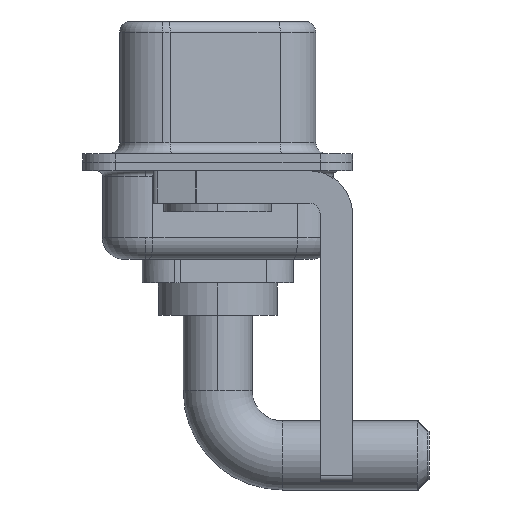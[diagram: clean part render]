
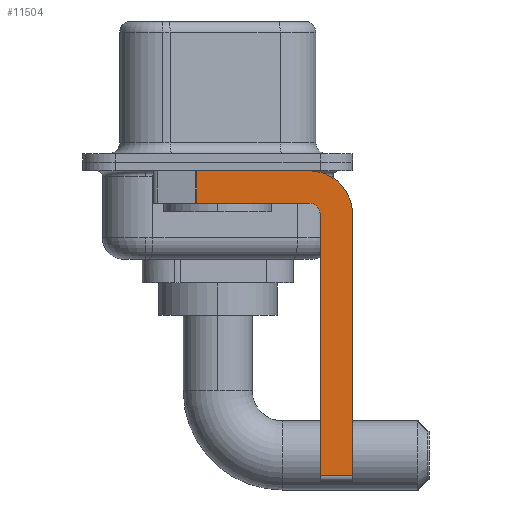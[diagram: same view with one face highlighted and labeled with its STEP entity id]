
A CAD part, left-side view. The second image highlights one B-rep face of the part: STEP entity #11504.
In plain terms, the highlighted planar face has unit normal (-1, 0, 0).
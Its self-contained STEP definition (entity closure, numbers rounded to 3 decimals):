
#90 = DIRECTION ( 'NONE',  ( 1., 0., 0. ) ) ;
#1001 = EDGE_CURVE ( 'NONE', #4662, #14181, #7622, .T. ) ;
#1189 = EDGE_CURVE ( 'NONE', #8029, #4716, #5484, .T. ) ;
#1194 = PLANE ( 'NONE',  #11478 ) ;
#1483 = CARTESIAN_POINT ( 'NONE',  ( -2.9, -4.25, -2.4 ) ) ;
#1550 = CARTESIAN_POINT ( 'NONE',  ( -2.9, -4.25, -2.4 ) ) ;
#1614 = CARTESIAN_POINT ( 'NONE',  ( -2.9, -4.25, -1.9 ) ) ;
#2068 = CARTESIAN_POINT ( 'NONE',  ( -2.9, 0.978, -1.9 ) ) ;
#2155 = CIRCLE ( 'NONE', #12160, 2. ) ;
#2481 = CARTESIAN_POINT ( 'NONE',  ( -2.9, 0.978, -0.4 ) ) ;
#3191 = CARTESIAN_POINT ( 'NONE',  ( -2.9, -4.75, -14.55 ) ) ;
#3294 = CARTESIAN_POINT ( 'NONE',  ( -2.9, -4.25, -0.4 ) ) ;
#3359 = CARTESIAN_POINT ( 'NONE',  ( -2.9, -4.75, -14.8 ) ) ;
#3788 = CARTESIAN_POINT ( 'NONE',  ( -2.9, -6.25, -2.4 ) ) ;
#3823 = EDGE_CURVE ( 'NONE', #8029, #11054, #7006, .T. ) ;
#3833 = CIRCLE ( 'NONE', #7467, 0.5 ) ;
#4075 = DIRECTION ( 'NONE',  ( 0., 1., 0. ) ) ;
#4662 = VERTEX_POINT ( 'NONE', #2481 ) ;
#4716 = VERTEX_POINT ( 'NONE', #11966 ) ;
#4869 = VERTEX_POINT ( 'NONE', #3788 ) ;
#4920 = EDGE_CURVE ( 'NONE', #11054, #5854, #3833, .T. ) ;
#4952 = EDGE_CURVE ( 'NONE', #4662, #5719, #13180, .T. ) ;
#5365 = ORIENTED_EDGE ( 'NONE', *, *, #5512, .F. ) ;
#5484 = LINE ( 'NONE', #8915, #11324 ) ;
#5512 = EDGE_CURVE ( 'NONE', #5854, #5719, #7645, .T. ) ;
#5719 = VERTEX_POINT ( 'NONE', #2068 ) ;
#5854 = VERTEX_POINT ( 'NONE', #13979 ) ;
#5855 = DIRECTION ( 'NONE',  ( 1., 0., 0. ) ) ;
#6202 = DIRECTION ( 'NONE',  ( 0., 0., -1. ) ) ;
#6381 = EDGE_CURVE ( 'NONE', #14181, #4869, #2155, .T. ) ;
#6847 = CARTESIAN_POINT ( 'NONE',  ( -2.9, -4.25, -2.4 ) ) ;
#7006 = LINE ( 'NONE', #3359, #7976 ) ;
#7363 = DIRECTION ( 'NONE',  ( 0., 0., -1. ) ) ;
#7467 = AXIS2_PLACEMENT_3D ( 'NONE', #1550, #11728, #14015 ) ;
#7622 = LINE ( 'NONE', #13445, #9769 ) ;
#7645 = LINE ( 'NONE', #1614, #8222 ) ;
#7976 = VECTOR ( 'NONE', #8086, 1000. ) ;
#8029 = VERTEX_POINT ( 'NONE', #3191 ) ;
#8086 = DIRECTION ( 'NONE',  ( 0., 0., 1. ) ) ;
#8222 = VECTOR ( 'NONE', #4075, 1000. ) ;
#8593 = ORIENTED_EDGE ( 'NONE', *, *, #1001, .F. ) ;
#8915 = CARTESIAN_POINT ( 'NONE',  ( -2.9, -4.25, -14.55 ) ) ;
#9021 = ORIENTED_EDGE ( 'NONE', *, *, #11549, .F. ) ;
#9769 = VECTOR ( 'NONE', #14422, 1000. ) ;
#10287 = DIRECTION ( 'NONE',  ( 0., -1., 0. ) ) ;
#10639 = VECTOR ( 'NONE', #6202, 1000. ) ;
#10672 = LINE ( 'NONE', #12047, #14400 ) ;
#11054 = VERTEX_POINT ( 'NONE', #11539 ) ;
#11249 = ORIENTED_EDGE ( 'NONE', *, *, #4952, .T. ) ;
#11324 = VECTOR ( 'NONE', #10287, 1000. ) ;
#11478 = AXIS2_PLACEMENT_3D ( 'NONE', #6847, #5855, #11523 ) ;
#11504 = ADVANCED_FACE ( 'NONE', ( #12813 ), #1194, .F. ) ;
#11523 = DIRECTION ( 'NONE',  ( 0., 0., -1. ) ) ;
#11539 = CARTESIAN_POINT ( 'NONE',  ( -2.9, -4.75, -2.4 ) ) ;
#11549 = EDGE_CURVE ( 'NONE', #4869, #4716, #10672, .T. ) ;
#11708 = ORIENTED_EDGE ( 'NONE', *, *, #1189, .T. ) ;
#11728 = DIRECTION ( 'NONE',  ( -1., 0., 0. ) ) ;
#11966 = CARTESIAN_POINT ( 'NONE',  ( -2.9, -6.25, -14.55 ) ) ;
#11977 = ORIENTED_EDGE ( 'NONE', *, *, #4920, .F. ) ;
#12026 = CARTESIAN_POINT ( 'NONE',  ( -2.9, 0.978, -1.9 ) ) ;
#12047 = CARTESIAN_POINT ( 'NONE',  ( -2.9, -6.25, -2.4 ) ) ;
#12160 = AXIS2_PLACEMENT_3D ( 'NONE', #1483, #90, #7363 ) ;
#12756 = ORIENTED_EDGE ( 'NONE', *, *, #6381, .F. ) ;
#12813 = FACE_OUTER_BOUND ( 'NONE', #12979, .T. ) ;
#12979 = EDGE_LOOP ( 'NONE', ( #8593, #11249, #5365, #11977, #13938, #11708, #9021, #12756 ) ) ;
#13180 = LINE ( 'NONE', #12026, #10639 ) ;
#13200 = DIRECTION ( 'NONE',  ( 0., 0., -1. ) ) ;
#13445 = CARTESIAN_POINT ( 'NONE',  ( -2.9, 3., -0.4 ) ) ;
#13938 = ORIENTED_EDGE ( 'NONE', *, *, #3823, .F. ) ;
#13979 = CARTESIAN_POINT ( 'NONE',  ( -2.9, -4.25, -1.9 ) ) ;
#14015 = DIRECTION ( 'NONE',  ( 0., 0., 1. ) ) ;
#14181 = VERTEX_POINT ( 'NONE', #3294 ) ;
#14400 = VECTOR ( 'NONE', #13200, 1000. ) ;
#14422 = DIRECTION ( 'NONE',  ( 0., -1., 0. ) ) ;
